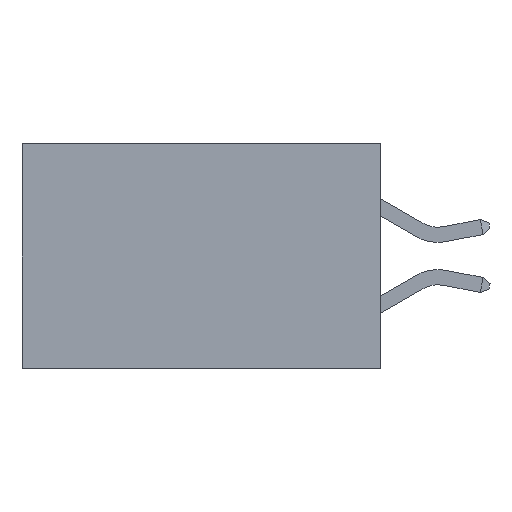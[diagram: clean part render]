
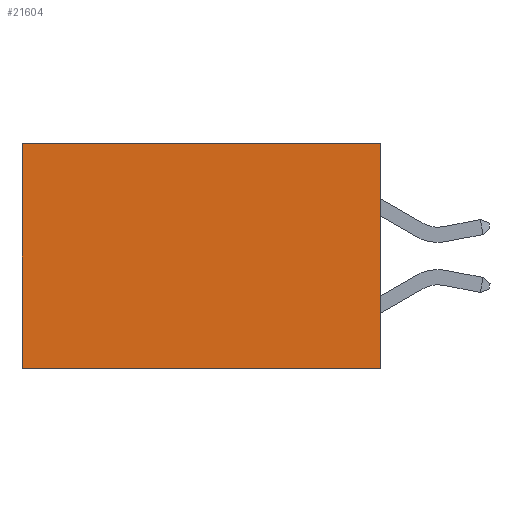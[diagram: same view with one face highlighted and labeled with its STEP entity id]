
A CAD part, left-side view. The second image highlights one B-rep face of the part: STEP entity #21604.
In plain terms, the highlighted planar face has unit normal (-1, 0, 0).
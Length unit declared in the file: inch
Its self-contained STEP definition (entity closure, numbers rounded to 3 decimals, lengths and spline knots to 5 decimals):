
#243 = CARTESIAN_POINT ( 'NONE',  ( 0.277, 0., -0.37 ) ) ;
#746 = VECTOR ( 'NONE', #17060, 39.37008 ) ;
#787 = CARTESIAN_POINT ( 'NONE',  ( 0.277, 0., 0. ) ) ;
#1371 = CARTESIAN_POINT ( 'NONE',  ( 0.277, 0.59, -0.37 ) ) ;
#3242 = EDGE_CURVE ( 'NONE', #17249, #13562, #29901, .T. ) ;
#4426 = VECTOR ( 'NONE', #10252, 39.37008 ) ;
#5277 = CARTESIAN_POINT ( 'NONE',  ( 0.277, 0., -0.37 ) ) ;
#5930 = LINE ( 'NONE', #24292, #6690 ) ;
#6690 = VECTOR ( 'NONE', #24188, 39.37008 ) ;
#9033 = ORIENTED_EDGE ( 'NONE', *, *, #26926, .F. ) ;
#10252 = DIRECTION ( 'NONE',  ( 0., 0., -1. ) ) ;
#10708 = CARTESIAN_POINT ( 'NONE',  ( 0.277, 0.59, -0.37 ) ) ;
#11448 = EDGE_LOOP ( 'NONE', ( #18654, #9033, #13373, #25106 ) ) ;
#11685 = PLANE ( 'NONE',  #17752 ) ;
#13249 = EDGE_CURVE ( 'NONE', #22689, #15251, #14314, .T. ) ;
#13373 = ORIENTED_EDGE ( 'NONE', *, *, #13249, .F. ) ;
#13562 = VERTEX_POINT ( 'NONE', #1371 ) ;
#14106 = DIRECTION ( 'NONE',  ( 1., 0., 0. ) ) ;
#14314 = LINE ( 'NONE', #243, #746 ) ;
#15172 = DIRECTION ( 'NONE',  ( 0., 1., 0. ) ) ;
#15251 = VERTEX_POINT ( 'NONE', #5277 ) ;
#16113 = LINE ( 'NONE', #29437, #28041 ) ;
#17060 = DIRECTION ( 'NONE',  ( 0., 0., -1. ) ) ;
#17249 = VERTEX_POINT ( 'NONE', #23724 ) ;
#17752 = AXIS2_PLACEMENT_3D ( 'NONE', #25960, #14106, #30767 ) ;
#18654 = ORIENTED_EDGE ( 'NONE', *, *, #3242, .T. ) ;
#18806 = FACE_OUTER_BOUND ( 'NONE', #11448, .T. ) ;
#21604 = ADVANCED_FACE ( 'NONE', ( #18806 ), #11685, .F. ) ;
#22689 = VERTEX_POINT ( 'NONE', #787 ) ;
#23724 = CARTESIAN_POINT ( 'NONE',  ( 0.277, 0.59, 0. ) ) ;
#24188 = DIRECTION ( 'NONE',  ( 0., 1., 0. ) ) ;
#24292 = CARTESIAN_POINT ( 'NONE',  ( 0.277, 0., 0. ) ) ;
#24508 = EDGE_CURVE ( 'NONE', #22689, #17249, #5930, .T. ) ;
#25106 = ORIENTED_EDGE ( 'NONE', *, *, #24508, .T. ) ;
#25960 = CARTESIAN_POINT ( 'NONE',  ( 0.277, 0., -0.37 ) ) ;
#26926 = EDGE_CURVE ( 'NONE', #15251, #13562, #16113, .T. ) ;
#28041 = VECTOR ( 'NONE', #15172, 39.37008 ) ;
#29437 = CARTESIAN_POINT ( 'NONE',  ( 0.277, 0., -0.37 ) ) ;
#29901 = LINE ( 'NONE', #10708, #4426 ) ;
#30767 = DIRECTION ( 'NONE',  ( 0., 0., -1. ) ) ;
